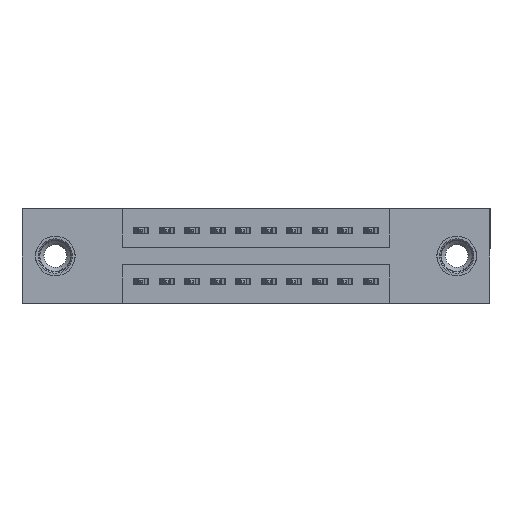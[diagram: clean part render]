
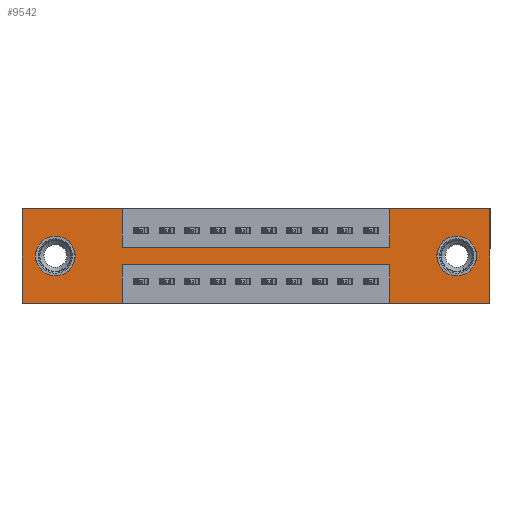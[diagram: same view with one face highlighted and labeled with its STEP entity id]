
A CAD part, front view. The second image highlights one B-rep face of the part: STEP entity #9542.
In plain terms, the highlighted planar face has unit normal (0, -1, 0).
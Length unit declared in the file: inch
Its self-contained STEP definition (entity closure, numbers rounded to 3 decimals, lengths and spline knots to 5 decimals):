
#132 = DIRECTION ( 'NONE',  ( 0., 0., 1. ) ) ;
#381 = DIRECTION ( 'NONE',  ( 0., 0., 1. ) ) ;
#490 = ORIENTED_EDGE ( 'NONE', *, *, #15316, .T. ) ;
#529 = ORIENTED_EDGE ( 'NONE', *, *, #9084, .F. ) ;
#732 = CARTESIAN_POINT ( 'NONE',  ( 0.3925, 0., -0.37 ) ) ;
#1120 = LINE ( 'NONE', #10655, #8222 ) ;
#1259 = FACE_OUTER_BOUND ( 'NONE', #16583, .T. ) ;
#1346 = LINE ( 'NONE', #9118, #14853 ) ;
#1540 = DIRECTION ( 'NONE',  ( 0., 1., 0. ) ) ;
#1670 = FACE_BOUND ( 'NONE', #15307, .T. ) ;
#1857 = ORIENTED_EDGE ( 'NONE', *, *, #12788, .T. ) ;
#1915 = DIRECTION ( 'NONE',  ( 1., 0., 0. ) ) ;
#2054 = DIRECTION ( 'NONE',  ( -1., 0., 0. ) ) ;
#2490 = LINE ( 'NONE', #9730, #2945 ) ;
#2661 = ORIENTED_EDGE ( 'NONE', *, *, #12050, .F. ) ;
#2792 = CARTESIAN_POINT ( 'NONE',  ( 0.3925, 0., 0. ) ) ;
#2945 = VECTOR ( 'NONE', #132, 39.37008 ) ;
#2982 = CARTESIAN_POINT ( 'NONE',  ( 0.3925, 0., 0. ) ) ;
#3280 = VERTEX_POINT ( 'NONE', #2982 ) ;
#3547 = LINE ( 'NONE', #6530, #13880 ) ;
#3615 = VECTOR ( 'NONE', #15879, 39.37008 ) ;
#3822 = VERTEX_POINT ( 'NONE', #4154 ) ;
#4154 = CARTESIAN_POINT ( 'NONE',  ( 1.4425, 0., -0.37 ) ) ;
#4315 = EDGE_CURVE ( 'NONE', #3822, #7734, #2490, .T. ) ;
#4471 = VECTOR ( 'NONE', #1915, 39.37008 ) ;
#4752 = EDGE_CURVE ( 'NONE', #13774, #7450, #16664, .T. ) ;
#4819 = ORIENTED_EDGE ( 'NONE', *, *, #12456, .F. ) ;
#4984 = VECTOR ( 'NONE', #11952, 39.37008 ) ;
#5429 = VECTOR ( 'NONE', #14340, 39.37008 ) ;
#5572 = CARTESIAN_POINT ( 'NONE',  ( 0.13, 0., -0.107 ) ) ;
#5604 = CARTESIAN_POINT ( 'NONE',  ( 1.4425, 0., -0.15 ) ) ;
#5822 = CARTESIAN_POINT ( 'NONE',  ( 1.835, 0., 0. ) ) ;
#5901 = VERTEX_POINT ( 'NONE', #6834 ) ;
#5999 = DIRECTION ( 'NONE',  ( 0., 0., -1. ) ) ;
#6015 = CIRCLE ( 'NONE', #16104, 0.078 ) ;
#6050 = CARTESIAN_POINT ( 'NONE',  ( 0.3925, 0., -0.15 ) ) ;
#6202 = EDGE_CURVE ( 'NONE', #7269, #15699, #1346, .T. ) ;
#6316 = CARTESIAN_POINT ( 'NONE',  ( 1.705, 0., -0.185 ) ) ;
#6398 = ORIENTED_EDGE ( 'NONE', *, *, #15983, .F. ) ;
#6493 = EDGE_CURVE ( 'NONE', #9229, #6944, #14635, .T. ) ;
#6530 = CARTESIAN_POINT ( 'NONE',  ( 0., 0., 0. ) ) ;
#6731 = EDGE_CURVE ( 'NONE', #8711, #5901, #14839, .T. ) ;
#6834 = CARTESIAN_POINT ( 'NONE',  ( 1.705, 0., -0.263 ) ) ;
#6944 = VERTEX_POINT ( 'NONE', #5572 ) ;
#7260 = DIRECTION ( 'NONE',  ( 0., 1., 0. ) ) ;
#7269 = VERTEX_POINT ( 'NONE', #732 ) ;
#7350 = CIRCLE ( 'NONE', #14415, 0.078 ) ;
#7450 = VERTEX_POINT ( 'NONE', #15449 ) ;
#7614 = DIRECTION ( 'NONE',  ( 0., 0., -1. ) ) ;
#7734 = VERTEX_POINT ( 'NONE', #12049 ) ;
#7820 = CARTESIAN_POINT ( 'NONE',  ( 1.835, 0., 0. ) ) ;
#7821 = AXIS2_PLACEMENT_3D ( 'NONE', #11134, #13694, #5999 ) ;
#7949 = VECTOR ( 'NONE', #13751, 39.37008 ) ;
#8222 = VECTOR ( 'NONE', #9370, 39.37008 ) ;
#8349 = FACE_BOUND ( 'NONE', #15520, .T. ) ;
#8376 = VERTEX_POINT ( 'NONE', #12189 ) ;
#8422 = DIRECTION ( 'NONE',  ( 0., 1., 0. ) ) ;
#8618 = DIRECTION ( 'NONE',  ( 0., 0., 1. ) ) ;
#8678 = CARTESIAN_POINT ( 'NONE',  ( 0.3925, 0., -0.22 ) ) ;
#8711 = VERTEX_POINT ( 'NONE', #9194 ) ;
#8754 = ORIENTED_EDGE ( 'NONE', *, *, #6493, .T. ) ;
#8885 = LINE ( 'NONE', #9270, #5429 ) ;
#9082 = ORIENTED_EDGE ( 'NONE', *, *, #12164, .F. ) ;
#9084 = EDGE_CURVE ( 'NONE', #8376, #3280, #11390, .T. ) ;
#9102 = CARTESIAN_POINT ( 'NONE',  ( 0.3925, 0., -0.22 ) ) ;
#9118 = CARTESIAN_POINT ( 'NONE',  ( 0., 0., -0.37 ) ) ;
#9155 = ORIENTED_EDGE ( 'NONE', *, *, #4752, .F. ) ;
#9194 = CARTESIAN_POINT ( 'NONE',  ( 1.705, 0., -0.107 ) ) ;
#9202 = VERTEX_POINT ( 'NONE', #15170 ) ;
#9220 = ORIENTED_EDGE ( 'NONE', *, *, #4315, .F. ) ;
#9229 = VERTEX_POINT ( 'NONE', #15230 ) ;
#9270 = CARTESIAN_POINT ( 'NONE',  ( 0.3925, 0., -0.37 ) ) ;
#9370 = DIRECTION ( 'NONE',  ( 0., 0., 1. ) ) ;
#9502 = CARTESIAN_POINT ( 'NONE',  ( 0.13, 0., -0.185 ) ) ;
#9542 = ADVANCED_FACE ( 'NONE', ( #8349, #1670, #1259 ), #12427, .T. ) ;
#9575 = EDGE_CURVE ( 'NONE', #11705, #13937, #10965, .T. ) ;
#9730 = CARTESIAN_POINT ( 'NONE',  ( 1.4425, 0., -0.37 ) ) ;
#9974 = LINE ( 'NONE', #8678, #13389 ) ;
#10130 = CARTESIAN_POINT ( 'NONE',  ( 0., 0., -0.37 ) ) ;
#10186 = ORIENTED_EDGE ( 'NONE', *, *, #11623, .F. ) ;
#10331 = ORIENTED_EDGE ( 'NONE', *, *, #6202, .F. ) ;
#10406 = DIRECTION ( 'NONE',  ( -1., 0., 0. ) ) ;
#10548 = LINE ( 'NONE', #13329, #3615 ) ;
#10655 = CARTESIAN_POINT ( 'NONE',  ( 1.4425, 0., 0. ) ) ;
#10785 = DIRECTION ( 'NONE',  ( 0., 0., 1. ) ) ;
#10865 = LINE ( 'NONE', #15064, #14654 ) ;
#10965 = LINE ( 'NONE', #6050, #7949 ) ;
#11134 = CARTESIAN_POINT ( 'NONE',  ( 0., 0., -0.37 ) ) ;
#11390 = LINE ( 'NONE', #14941, #4471 ) ;
#11408 = ORIENTED_EDGE ( 'NONE', *, *, #9575, .F. ) ;
#11515 = VERTEX_POINT ( 'NONE', #9102 ) ;
#11585 = AXIS2_PLACEMENT_3D ( 'NONE', #6316, #15315, #7614 ) ;
#11623 = EDGE_CURVE ( 'NONE', #11515, #7269, #8885, .T. ) ;
#11700 = ORIENTED_EDGE ( 'NONE', *, *, #13330, .F. ) ;
#11705 = VERTEX_POINT ( 'NONE', #14562 ) ;
#11905 = AXIS2_PLACEMENT_3D ( 'NONE', #16077, #8422, #381 ) ;
#11952 = DIRECTION ( 'NONE',  ( 0., 0., -1. ) ) ;
#12049 = CARTESIAN_POINT ( 'NONE',  ( 1.4425, 0., -0.22 ) ) ;
#12050 = EDGE_CURVE ( 'NONE', #9202, #13774, #3547, .T. ) ;
#12164 = EDGE_CURVE ( 'NONE', #3280, #11705, #12692, .T. ) ;
#12189 = CARTESIAN_POINT ( 'NONE',  ( 0., 0., 0. ) ) ;
#12427 = PLANE ( 'NONE',  #7821 ) ;
#12456 = EDGE_CURVE ( 'NONE', #15699, #8376, #10865, .T. ) ;
#12692 = LINE ( 'NONE', #2792, #4984 ) ;
#12698 = ORIENTED_EDGE ( 'NONE', *, *, #15360, .F. ) ;
#12788 = EDGE_CURVE ( 'NONE', #6944, #9229, #6015, .T. ) ;
#13313 = VECTOR ( 'NONE', #14858, 39.37008 ) ;
#13329 = CARTESIAN_POINT ( 'NONE',  ( 0., 0., -0.37 ) ) ;
#13330 = EDGE_CURVE ( 'NONE', #13937, #9202, #1120, .T. ) ;
#13389 = VECTOR ( 'NONE', #2054, 39.37008 ) ;
#13694 = DIRECTION ( 'NONE',  ( 0., -1., 0. ) ) ;
#13751 = DIRECTION ( 'NONE',  ( 1., 0., 0. ) ) ;
#13774 = VERTEX_POINT ( 'NONE', #7820 ) ;
#13880 = VECTOR ( 'NONE', #15517, 39.37008 ) ;
#13937 = VERTEX_POINT ( 'NONE', #5604 ) ;
#14340 = DIRECTION ( 'NONE',  ( 0., 0., -1. ) ) ;
#14415 = AXIS2_PLACEMENT_3D ( 'NONE', #14961, #7260, #16222 ) ;
#14562 = CARTESIAN_POINT ( 'NONE',  ( 0.3925, 0., -0.15 ) ) ;
#14635 = CIRCLE ( 'NONE', #11905, 0.078 ) ;
#14654 = VECTOR ( 'NONE', #8618, 39.37008 ) ;
#14839 = CIRCLE ( 'NONE', #11585, 0.078 ) ;
#14853 = VECTOR ( 'NONE', #10406, 39.37008 ) ;
#14858 = DIRECTION ( 'NONE',  ( 0., 0., -1. ) ) ;
#14941 = CARTESIAN_POINT ( 'NONE',  ( 0., 0., 0. ) ) ;
#14961 = CARTESIAN_POINT ( 'NONE',  ( 1.705, 0., -0.185 ) ) ;
#15064 = CARTESIAN_POINT ( 'NONE',  ( 0., 0., 0. ) ) ;
#15170 = CARTESIAN_POINT ( 'NONE',  ( 1.4425, 0., 0. ) ) ;
#15230 = CARTESIAN_POINT ( 'NONE',  ( 0.13, 0., -0.263 ) ) ;
#15307 = EDGE_LOOP ( 'NONE', ( #1857, #8754 ) ) ;
#15315 = DIRECTION ( 'NONE',  ( 0., 1., 0. ) ) ;
#15316 = EDGE_CURVE ( 'NONE', #5901, #8711, #7350, .T. ) ;
#15360 = EDGE_CURVE ( 'NONE', #7734, #11515, #9974, .T. ) ;
#15449 = CARTESIAN_POINT ( 'NONE',  ( 1.835, 0., -0.37 ) ) ;
#15517 = DIRECTION ( 'NONE',  ( 1., 0., 0. ) ) ;
#15520 = EDGE_LOOP ( 'NONE', ( #16103, #490 ) ) ;
#15699 = VERTEX_POINT ( 'NONE', #10130 ) ;
#15879 = DIRECTION ( 'NONE',  ( -1., 0., 0. ) ) ;
#15983 = EDGE_CURVE ( 'NONE', #7450, #3822, #10548, .T. ) ;
#16077 = CARTESIAN_POINT ( 'NONE',  ( 0.13, 0., -0.185 ) ) ;
#16103 = ORIENTED_EDGE ( 'NONE', *, *, #6731, .T. ) ;
#16104 = AXIS2_PLACEMENT_3D ( 'NONE', #9502, #1540, #10785 ) ;
#16222 = DIRECTION ( 'NONE',  ( 0., 0., -1. ) ) ;
#16583 = EDGE_LOOP ( 'NONE', ( #10186, #12698, #9220, #6398, #9155, #2661, #11700, #11408, #9082, #529, #4819, #10331 ) ) ;
#16664 = LINE ( 'NONE', #5822, #13313 ) ;
